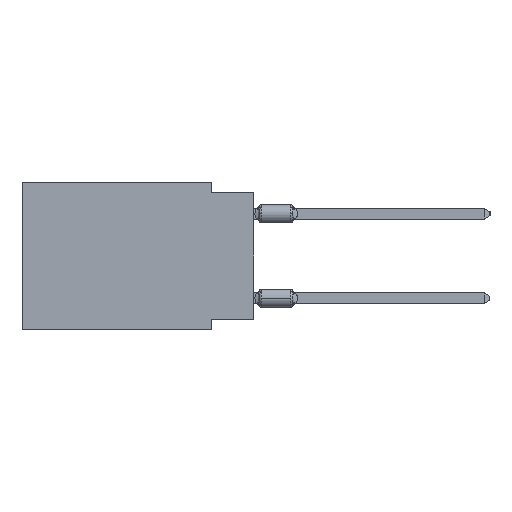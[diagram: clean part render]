
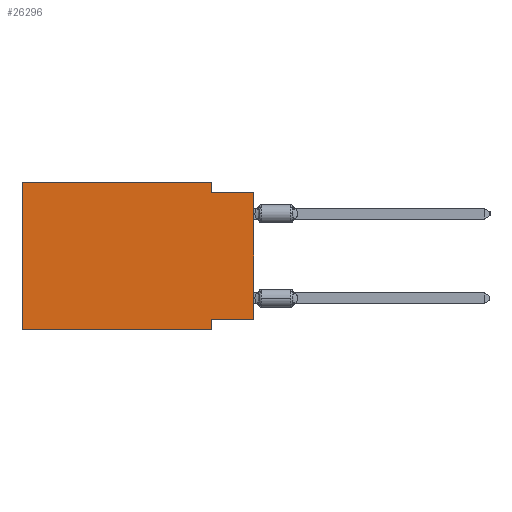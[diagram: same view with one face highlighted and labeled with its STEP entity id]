
A CAD part, left-side view. The second image highlights one B-rep face of the part: STEP entity #26296.
In plain terms, the highlighted planar face has unit normal (-1, 0, 0).
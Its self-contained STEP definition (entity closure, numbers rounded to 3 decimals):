
#1856 = CARTESIAN_POINT ( 'NONE',  ( 0., 0., -0.635 ) ) ;
#2029 = CARTESIAN_POINT ( 'NONE',  ( 0., 0., -8.255 ) ) ;
#2229 = CARTESIAN_POINT ( 'NONE',  ( 0., 2.54, -8.89 ) ) ;
#2262 = EDGE_CURVE ( 'NONE', #66208, #34915, #12047, .T. ) ;
#2652 = AXIS2_PLACEMENT_3D ( 'NONE', #33512, #54575, #29394 ) ;
#3337 = EDGE_LOOP ( 'NONE', ( #19591, #20322, #38753, #40207, #7964, #65046, #26778, #25469 ) ) ;
#5305 = VECTOR ( 'NONE', #12587, 1000. ) ;
#6943 = DIRECTION ( 'NONE',  ( 0., -1., 0. ) ) ;
#7074 = CARTESIAN_POINT ( 'NONE',  ( 0., 13.97, -8.89 ) ) ;
#7785 = VERTEX_POINT ( 'NONE', #51269 ) ;
#7964 = ORIENTED_EDGE ( 'NONE', *, *, #51054, .F. ) ;
#8557 = CARTESIAN_POINT ( 'NONE',  ( 0., 2.54, 0. ) ) ;
#9057 = CARTESIAN_POINT ( 'NONE',  ( 0., 0., 0. ) ) ;
#9084 = VECTOR ( 'NONE', #49201, 1000. ) ;
#9233 = CARTESIAN_POINT ( 'NONE',  ( 0., 13.97, 0. ) ) ;
#10242 = VERTEX_POINT ( 'NONE', #46723 ) ;
#12047 = LINE ( 'NONE', #32147, #46818 ) ;
#12587 = DIRECTION ( 'NONE',  ( 0., 1., 0. ) ) ;
#12772 = LINE ( 'NONE', #24263, #39184 ) ;
#12912 = LINE ( 'NONE', #2029, #5305 ) ;
#13406 = PLANE ( 'NONE',  #2652 ) ;
#13981 = LINE ( 'NONE', #9233, #60582 ) ;
#14671 = LINE ( 'NONE', #8557, #49422 ) ;
#17769 = CARTESIAN_POINT ( 'NONE',  ( 0., 13.97, 0. ) ) ;
#18452 = EDGE_CURVE ( 'NONE', #34056, #10242, #14671, .T. ) ;
#18962 = LINE ( 'NONE', #66603, #55123 ) ;
#19591 = ORIENTED_EDGE ( 'NONE', *, *, #50260, .T. ) ;
#19961 = DIRECTION ( 'NONE',  ( 0., -1., 0. ) ) ;
#20322 = ORIENTED_EDGE ( 'NONE', *, *, #20920, .F. ) ;
#20920 = EDGE_CURVE ( 'NONE', #10242, #25403, #18962, .T. ) ;
#21783 = CARTESIAN_POINT ( 'NONE',  ( 0., 2.54, 0. ) ) ;
#24263 = CARTESIAN_POINT ( 'NONE',  ( 0., 13.97, 0. ) ) ;
#25403 = VERTEX_POINT ( 'NONE', #1856 ) ;
#25469 = ORIENTED_EDGE ( 'NONE', *, *, #52564, .F. ) ;
#26296 = ADVANCED_FACE ( 'NONE', ( #49146 ), #13406, .F. ) ;
#26778 = ORIENTED_EDGE ( 'NONE', *, *, #59628, .F. ) ;
#29394 = DIRECTION ( 'NONE',  ( 0., 0., -1. ) ) ;
#29824 = LINE ( 'NONE', #9057, #64274 ) ;
#32147 = CARTESIAN_POINT ( 'NONE',  ( 0., 13.97, -8.89 ) ) ;
#33512 = CARTESIAN_POINT ( 'NONE',  ( 0., 13.97, 0. ) ) ;
#34056 = VERTEX_POINT ( 'NONE', #21783 ) ;
#34915 = VERTEX_POINT ( 'NONE', #48456 ) ;
#36272 = DIRECTION ( 'NONE',  ( 0., 0., 1. ) ) ;
#36413 = VERTEX_POINT ( 'NONE', #37511 ) ;
#37511 = CARTESIAN_POINT ( 'NONE',  ( 0., 2.54, -8.255 ) ) ;
#37650 = VERTEX_POINT ( 'NONE', #17769 ) ;
#38753 = ORIENTED_EDGE ( 'NONE', *, *, #18452, .F. ) ;
#39184 = VECTOR ( 'NONE', #45314, 1000. ) ;
#40207 = ORIENTED_EDGE ( 'NONE', *, *, #45634, .F. ) ;
#45314 = DIRECTION ( 'NONE',  ( 0., -1., 0. ) ) ;
#45610 = DIRECTION ( 'NONE',  ( 0., 0., 1. ) ) ;
#45634 = EDGE_CURVE ( 'NONE', #37650, #34056, #12772, .T. ) ;
#46723 = CARTESIAN_POINT ( 'NONE',  ( 0., 2.54, -0.635 ) ) ;
#46818 = VECTOR ( 'NONE', #6943, 1000. ) ;
#48456 = CARTESIAN_POINT ( 'NONE',  ( 0., 2.54, -8.89 ) ) ;
#49146 = FACE_OUTER_BOUND ( 'NONE', #3337, .T. ) ;
#49201 = DIRECTION ( 'NONE',  ( 0., 0., -1. ) ) ;
#49422 = VECTOR ( 'NONE', #61986, 1000. ) ;
#50260 = EDGE_CURVE ( 'NONE', #7785, #25403, #29824, .T. ) ;
#51054 = EDGE_CURVE ( 'NONE', #66208, #37650, #13981, .T. ) ;
#51269 = CARTESIAN_POINT ( 'NONE',  ( 0., 0., -8.255 ) ) ;
#52564 = EDGE_CURVE ( 'NONE', #7785, #36413, #12912, .T. ) ;
#54575 = DIRECTION ( 'NONE',  ( 1., 0., 0. ) ) ;
#55123 = VECTOR ( 'NONE', #19961, 1000. ) ;
#59397 = LINE ( 'NONE', #2229, #9084 ) ;
#59628 = EDGE_CURVE ( 'NONE', #36413, #34915, #59397, .T. ) ;
#60582 = VECTOR ( 'NONE', #45610, 1000. ) ;
#61986 = DIRECTION ( 'NONE',  ( 0., 0., -1. ) ) ;
#64274 = VECTOR ( 'NONE', #36272, 1000. ) ;
#65046 = ORIENTED_EDGE ( 'NONE', *, *, #2262, .T. ) ;
#66208 = VERTEX_POINT ( 'NONE', #7074 ) ;
#66603 = CARTESIAN_POINT ( 'NONE',  ( 0., 0., -0.635 ) ) ;
